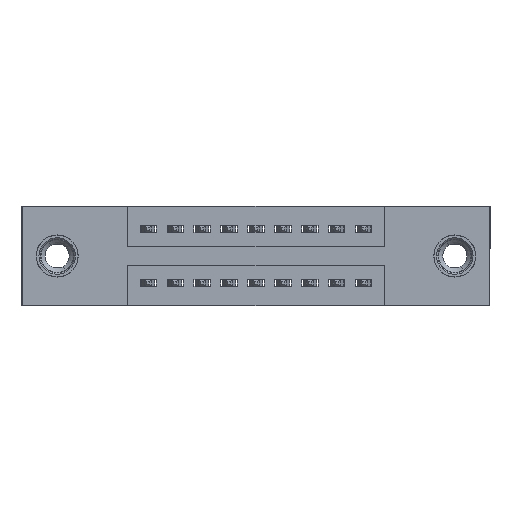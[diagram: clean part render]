
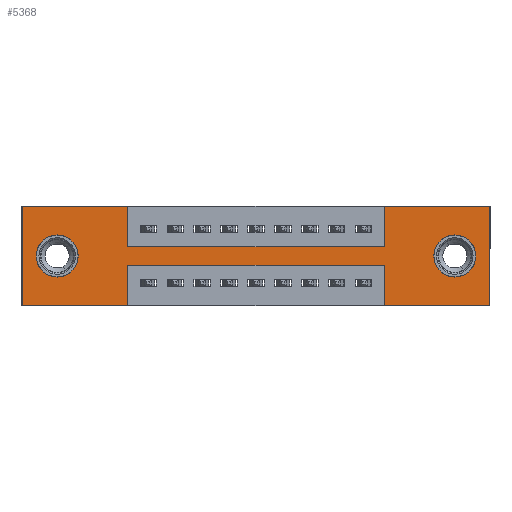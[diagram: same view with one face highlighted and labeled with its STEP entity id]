
A CAD part, front view. The second image highlights one B-rep face of the part: STEP entity #5368.
In plain terms, the highlighted planar face has unit normal (0, -1, 0).
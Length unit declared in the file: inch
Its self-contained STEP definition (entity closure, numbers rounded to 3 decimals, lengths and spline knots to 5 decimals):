
#141 = VECTOR ( 'NONE', #1513, 39.37008 ) ;
#292 = DIRECTION ( 'NONE',  ( 0., 0., 1. ) ) ;
#308 = LINE ( 'NONE', #7293, #3080 ) ;
#370 = ORIENTED_EDGE ( 'NONE', *, *, #11995, .T. ) ;
#446 = VECTOR ( 'NONE', #4512, 39.37008 ) ;
#574 = DIRECTION ( 'NONE',  ( 1., 0., 0. ) ) ;
#835 = DIRECTION ( 'NONE',  ( 0., 0., -1. ) ) ;
#836 = ORIENTED_EDGE ( 'NONE', *, *, #12245, .F. ) ;
#1231 = DIRECTION ( 'NONE',  ( 0., 1., 0. ) ) ;
#1320 = CARTESIAN_POINT ( 'NONE',  ( 0., 0., 0. ) ) ;
#1354 = CARTESIAN_POINT ( 'NONE',  ( 1.3425, 0., -0.15 ) ) ;
#1497 = CARTESIAN_POINT ( 'NONE',  ( 0.3925, 0., -0.15 ) ) ;
#1505 = LINE ( 'NONE', #1497, #12287 ) ;
#1513 = DIRECTION ( 'NONE',  ( -1., 0., 0. ) ) ;
#1611 = ORIENTED_EDGE ( 'NONE', *, *, #12845, .T. ) ;
#1786 = CARTESIAN_POINT ( 'NONE',  ( 1.605, 0., -0.107 ) ) ;
#1836 = VERTEX_POINT ( 'NONE', #11241 ) ;
#1988 = DIRECTION ( 'NONE',  ( 0., 0., -1. ) ) ;
#2047 = EDGE_CURVE ( 'NONE', #5396, #5531, #1505, .T. ) ;
#2136 = VERTEX_POINT ( 'NONE', #2780 ) ;
#2153 = ORIENTED_EDGE ( 'NONE', *, *, #11679, .F. ) ;
#2229 = ORIENTED_EDGE ( 'NONE', *, *, #12329, .T. ) ;
#2581 = CARTESIAN_POINT ( 'NONE',  ( 1.735, 0., -0.37 ) ) ;
#2780 = CARTESIAN_POINT ( 'NONE',  ( 0.13, 0., -0.107 ) ) ;
#2823 = VERTEX_POINT ( 'NONE', #1786 ) ;
#2919 = EDGE_LOOP ( 'NONE', ( #2229, #1611 ) ) ;
#2991 = ORIENTED_EDGE ( 'NONE', *, *, #11988, .F. ) ;
#3080 = VECTOR ( 'NONE', #1988, 39.37008 ) ;
#3125 = VECTOR ( 'NONE', #574, 39.37008 ) ;
#3135 = PLANE ( 'NONE',  #3290 ) ;
#3195 = CARTESIAN_POINT ( 'NONE',  ( 1.3425, 0., -0.37 ) ) ;
#3290 = AXIS2_PLACEMENT_3D ( 'NONE', #4276, #12431, #6325 ) ;
#3388 = CARTESIAN_POINT ( 'NONE',  ( 0.3925, 0., -0.37 ) ) ;
#3464 = EDGE_CURVE ( 'NONE', #3570, #7484, #5593, .T. ) ;
#3570 = VERTEX_POINT ( 'NONE', #7239 ) ;
#3790 = CARTESIAN_POINT ( 'NONE',  ( 0., 0., -0.37 ) ) ;
#3864 = LINE ( 'NONE', #7371, #11385 ) ;
#3946 = VECTOR ( 'NONE', #12885, 39.37008 ) ;
#4028 = AXIS2_PLACEMENT_3D ( 'NONE', #13407, #7335, #835 ) ;
#4114 = EDGE_LOOP ( 'NONE', ( #8305, #370 ) ) ;
#4276 = CARTESIAN_POINT ( 'NONE',  ( 0., 0., -0.37 ) ) ;
#4375 = VERTEX_POINT ( 'NONE', #13553 ) ;
#4430 = LINE ( 'NONE', #1320, #6827 ) ;
#4512 = DIRECTION ( 'NONE',  ( -1., 0., 0. ) ) ;
#4658 = ORIENTED_EDGE ( 'NONE', *, *, #3464, .F. ) ;
#4665 = AXIS2_PLACEMENT_3D ( 'NONE', #7680, #1231, #8692 ) ;
#4690 = CARTESIAN_POINT ( 'NONE',  ( 0.3925, 0., 0. ) ) ;
#4694 = ORIENTED_EDGE ( 'NONE', *, *, #12404, .F. ) ;
#4816 = ORIENTED_EDGE ( 'NONE', *, *, #10252, .F. ) ;
#4872 = LINE ( 'NONE', #3195, #9947 ) ;
#4918 = CARTESIAN_POINT ( 'NONE',  ( 0., 0., 0. ) ) ;
#4919 = FACE_BOUND ( 'NONE', #4114, .T. ) ;
#5368 = ADVANCED_FACE ( 'NONE', ( #4919, #6989, #12387 ), #3135, .T. ) ;
#5369 = VECTOR ( 'NONE', #9003, 39.37008 ) ;
#5396 = VERTEX_POINT ( 'NONE', #10613 ) ;
#5496 = ORIENTED_EDGE ( 'NONE', *, *, #11650, .F. ) ;
#5531 = VERTEX_POINT ( 'NONE', #1354 ) ;
#5593 = LINE ( 'NONE', #8132, #3125 ) ;
#6060 = CARTESIAN_POINT ( 'NONE',  ( 1.605, 0., -0.185 ) ) ;
#6207 = VERTEX_POINT ( 'NONE', #2581 ) ;
#6210 = VERTEX_POINT ( 'NONE', #12896 ) ;
#6325 = DIRECTION ( 'NONE',  ( 0., 0., -1. ) ) ;
#6504 = CARTESIAN_POINT ( 'NONE',  ( 1.3425, 0., -0.37 ) ) ;
#6687 = LINE ( 'NONE', #9809, #3946 ) ;
#6694 = DIRECTION ( 'NONE',  ( 0., 0., -1. ) ) ;
#6827 = VECTOR ( 'NONE', #10813, 39.37008 ) ;
#6875 = DIRECTION ( 'NONE',  ( 0., 1., 0. ) ) ;
#6989 = FACE_BOUND ( 'NONE', #2919, .T. ) ;
#7107 = DIRECTION ( 'NONE',  ( 0., 0., -1. ) ) ;
#7239 = CARTESIAN_POINT ( 'NONE',  ( 0., 0., 0. ) ) ;
#7259 = ORIENTED_EDGE ( 'NONE', *, *, #9401, .F. ) ;
#7293 = CARTESIAN_POINT ( 'NONE',  ( 0.3925, 0., 0. ) ) ;
#7300 = LINE ( 'NONE', #9752, #9992 ) ;
#7335 = DIRECTION ( 'NONE',  ( 0., 1., 0. ) ) ;
#7371 = CARTESIAN_POINT ( 'NONE',  ( 0., 0., -0.37 ) ) ;
#7388 = EDGE_CURVE ( 'NONE', #6207, #10665, #9019, .T. ) ;
#7459 = EDGE_LOOP ( 'NONE', ( #836, #4816, #10441, #8134, #2153, #5496, #7259, #8677, #2991, #4658, #4694, #8835 ) ) ;
#7484 = VERTEX_POINT ( 'NONE', #4690 ) ;
#7621 = VERTEX_POINT ( 'NONE', #3790 ) ;
#7680 = CARTESIAN_POINT ( 'NONE',  ( 0.13, 0., -0.185 ) ) ;
#7861 = LINE ( 'NONE', #13636, #9906 ) ;
#7886 = CARTESIAN_POINT ( 'NONE',  ( 0.3925, 0., -0.22 ) ) ;
#7896 = DIRECTION ( 'NONE',  ( 1., 0., 0. ) ) ;
#7906 = CARTESIAN_POINT ( 'NONE',  ( 0.3925, 0., -0.22 ) ) ;
#8096 = LINE ( 'NONE', #4918, #5369 ) ;
#8132 = CARTESIAN_POINT ( 'NONE',  ( 0., 0., 0. ) ) ;
#8134 = ORIENTED_EDGE ( 'NONE', *, *, #7388, .F. ) ;
#8138 = EDGE_CURVE ( 'NONE', #10665, #11077, #4872, .T. ) ;
#8240 = VERTEX_POINT ( 'NONE', #3388 ) ;
#8305 = ORIENTED_EDGE ( 'NONE', *, *, #10378, .T. ) ;
#8427 = VERTEX_POINT ( 'NONE', #12913 ) ;
#8597 = DIRECTION ( 'NONE',  ( 0., 0., 1. ) ) ;
#8677 = ORIENTED_EDGE ( 'NONE', *, *, #2047, .F. ) ;
#8692 = DIRECTION ( 'NONE',  ( 0., 0., 1. ) ) ;
#8835 = ORIENTED_EDGE ( 'NONE', *, *, #13690, .F. ) ;
#9003 = DIRECTION ( 'NONE',  ( 0., 0., 1. ) ) ;
#9019 = LINE ( 'NONE', #13614, #446 ) ;
#9094 = VERTEX_POINT ( 'NONE', #7886 ) ;
#9269 = AXIS2_PLACEMENT_3D ( 'NONE', #12965, #6875, #292 ) ;
#9401 = EDGE_CURVE ( 'NONE', #5531, #4375, #7861, .T. ) ;
#9524 = AXIS2_PLACEMENT_3D ( 'NONE', #6060, #13184, #7107 ) ;
#9752 = CARTESIAN_POINT ( 'NONE',  ( 0.3925, 0., -0.37 ) ) ;
#9809 = CARTESIAN_POINT ( 'NONE',  ( 1.735, 0., 0. ) ) ;
#9906 = VECTOR ( 'NONE', #8597, 39.37008 ) ;
#9947 = VECTOR ( 'NONE', #11371, 39.37008 ) ;
#9992 = VECTOR ( 'NONE', #6694, 39.37008 ) ;
#10252 = EDGE_CURVE ( 'NONE', #11077, #9094, #13537, .T. ) ;
#10378 = EDGE_CURVE ( 'NONE', #2823, #6210, #12264, .T. ) ;
#10441 = ORIENTED_EDGE ( 'NONE', *, *, #8138, .F. ) ;
#10613 = CARTESIAN_POINT ( 'NONE',  ( 0.3925, 0., -0.15 ) ) ;
#10665 = VERTEX_POINT ( 'NONE', #6504 ) ;
#10813 = DIRECTION ( 'NONE',  ( 1., 0., 0. ) ) ;
#10985 = CIRCLE ( 'NONE', #4028, 0.078 ) ;
#11077 = VERTEX_POINT ( 'NONE', #12994 ) ;
#11241 = CARTESIAN_POINT ( 'NONE',  ( 1.735, 0., 0. ) ) ;
#11371 = DIRECTION ( 'NONE',  ( 0., 0., 1. ) ) ;
#11385 = VECTOR ( 'NONE', #11446, 39.37008 ) ;
#11446 = DIRECTION ( 'NONE',  ( -1., 0., 0. ) ) ;
#11650 = EDGE_CURVE ( 'NONE', #4375, #1836, #4430, .T. ) ;
#11679 = EDGE_CURVE ( 'NONE', #1836, #6207, #6687, .T. ) ;
#11988 = EDGE_CURVE ( 'NONE', #7484, #5396, #308, .T. ) ;
#11995 = EDGE_CURVE ( 'NONE', #6210, #2823, #10985, .T. ) ;
#12063 = CIRCLE ( 'NONE', #9269, 0.078 ) ;
#12245 = EDGE_CURVE ( 'NONE', #9094, #8240, #7300, .T. ) ;
#12264 = CIRCLE ( 'NONE', #9524, 0.078 ) ;
#12287 = VECTOR ( 'NONE', #7896, 39.37008 ) ;
#12329 = EDGE_CURVE ( 'NONE', #2136, #8427, #12063, .T. ) ;
#12387 = FACE_OUTER_BOUND ( 'NONE', #7459, .T. ) ;
#12404 = EDGE_CURVE ( 'NONE', #7621, #3570, #8096, .T. ) ;
#12431 = DIRECTION ( 'NONE',  ( 0., -1., 0. ) ) ;
#12845 = EDGE_CURVE ( 'NONE', #8427, #2136, #13469, .T. ) ;
#12885 = DIRECTION ( 'NONE',  ( 0., 0., -1. ) ) ;
#12896 = CARTESIAN_POINT ( 'NONE',  ( 1.605, 0., -0.263 ) ) ;
#12913 = CARTESIAN_POINT ( 'NONE',  ( 0.13, 0., -0.263 ) ) ;
#12965 = CARTESIAN_POINT ( 'NONE',  ( 0.13, 0., -0.185 ) ) ;
#12994 = CARTESIAN_POINT ( 'NONE',  ( 1.3425, 0., -0.22 ) ) ;
#13184 = DIRECTION ( 'NONE',  ( 0., 1., 0. ) ) ;
#13407 = CARTESIAN_POINT ( 'NONE',  ( 1.605, 0., -0.185 ) ) ;
#13469 = CIRCLE ( 'NONE', #4665, 0.078 ) ;
#13537 = LINE ( 'NONE', #7906, #141 ) ;
#13553 = CARTESIAN_POINT ( 'NONE',  ( 1.3425, 0., 0. ) ) ;
#13614 = CARTESIAN_POINT ( 'NONE',  ( 0., 0., -0.37 ) ) ;
#13636 = CARTESIAN_POINT ( 'NONE',  ( 1.3425, 0., 0. ) ) ;
#13690 = EDGE_CURVE ( 'NONE', #8240, #7621, #3864, .T. ) ;
